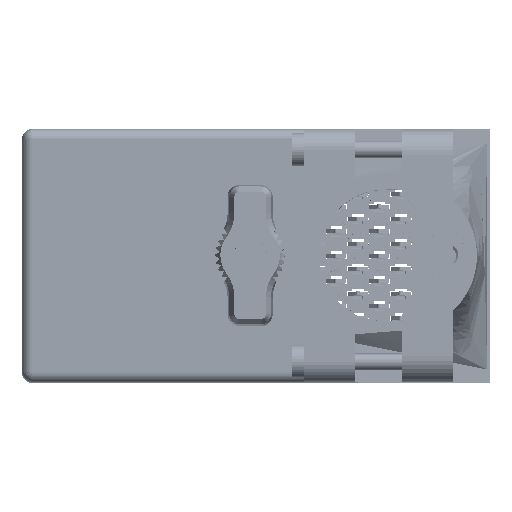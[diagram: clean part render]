
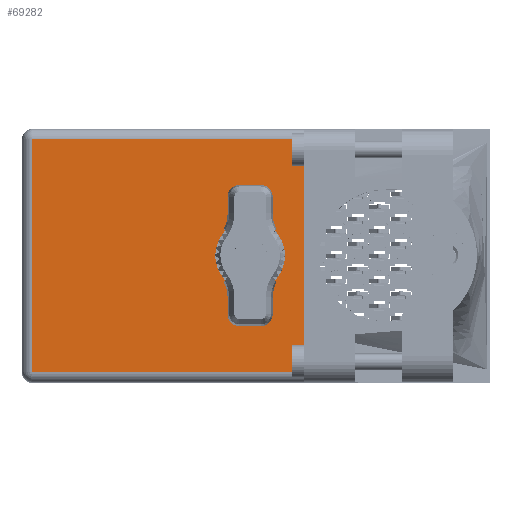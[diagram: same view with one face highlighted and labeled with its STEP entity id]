
A CAD part, top view. The second image highlights one B-rep face of the part: STEP entity #69282.
In plain terms, the highlighted face is planar.
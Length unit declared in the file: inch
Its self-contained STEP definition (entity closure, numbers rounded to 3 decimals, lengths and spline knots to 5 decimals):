
#1304 = ORIENTED_EDGE ( 'NONE', *, *, #88833, .F. ) ;
#4832 = DIRECTION ( 'NONE',  ( 0., 1., 0. ) ) ;
#9601 = VECTOR ( 'NONE', #106246, 39.37008 ) ;
#10069 = EDGE_CURVE ( 'NONE', #51063, #36797, #83982, .T. ) ;
#12342 = DIRECTION ( 'NONE',  ( 0., 1., 0. ) ) ;
#13008 = DIRECTION ( 'NONE',  ( 0., 0., 1. ) ) ;
#14986 = VERTEX_POINT ( 'NONE', #34446 ) ;
#15195 = CARTESIAN_POINT ( 'NONE',  ( 0., 1.93, -0.17 ) ) ;
#22111 = AXIS2_PLACEMENT_3D ( 'NONE', #31059, #4832, #13008 ) ;
#22613 = ORIENTED_EDGE ( 'NONE', *, *, #36865, .T. ) ;
#22828 = CARTESIAN_POINT ( 'NONE',  ( -1.3775, 1.93, -0.703 ) ) ;
#27226 = DIRECTION ( 'NONE',  ( 0., 0., 1. ) ) ;
#31059 = CARTESIAN_POINT ( 'NONE',  ( 0., 1.93, 0. ) ) ;
#33357 = EDGE_CURVE ( 'NONE', #52219, #81480, #93656, .T. ) ;
#34446 = CARTESIAN_POINT ( 'NONE',  ( 0.3275, 1.93, 0.703 ) ) ;
#34911 = VECTOR ( 'NONE', #67939, 39.37008 ) ;
#35451 = EDGE_LOOP ( 'NONE', ( #1304, #92665 ) ) ;
#36797 = VERTEX_POINT ( 'NONE', #104232 ) ;
#36865 = EDGE_CURVE ( 'NONE', #115911, #14986, #96219, .T. ) ;
#40876 = CIRCLE ( 'NONE', #74702, 0.17 ) ;
#41959 = DIRECTION ( 'NONE',  ( 1., 0., 0. ) ) ;
#43500 = ORIENTED_EDGE ( 'NONE', *, *, #45026, .T. ) ;
#45026 = EDGE_CURVE ( 'NONE', #81480, #115911, #51684, .T. ) ;
#45258 = DIRECTION ( 'NONE',  ( 0., 1., 0. ) ) ;
#48492 = VECTOR ( 'NONE', #107899, 39.37008 ) ;
#51063 = VERTEX_POINT ( 'NONE', #15195 ) ;
#51684 = LINE ( 'NONE', #105497, #9601 ) ;
#52219 = VERTEX_POINT ( 'NONE', #72164 ) ;
#55409 = AXIS2_PLACEMENT_3D ( 'NONE', #84063, #12342, #75034 ) ;
#55455 = FACE_BOUND ( 'NONE', #35451, .T. ) ;
#63740 = CARTESIAN_POINT ( 'NONE',  ( 0.3275, 1.93, -0.765 ) ) ;
#67939 = DIRECTION ( 'NONE',  ( -1., 0., 0. ) ) ;
#69282 = ADVANCED_FACE ( 'NONE', ( #79278, #55455 ), #75411, .T. ) ;
#72164 = CARTESIAN_POINT ( 'NONE',  ( 0.3275, 1.93, -0.703 ) ) ;
#74702 = AXIS2_PLACEMENT_3D ( 'NONE', #88771, #45258, #27226 ) ;
#75034 = DIRECTION ( 'NONE',  ( -1., 0., 0. ) ) ;
#75411 = PLANE ( 'NONE',  #55409 ) ;
#78103 = EDGE_LOOP ( 'NONE', ( #43500, #22613, #99815, #103140 ) ) ;
#79278 = FACE_OUTER_BOUND ( 'NONE', #78103, .T. ) ;
#80683 = LINE ( 'NONE', #63740, #48492 ) ;
#81480 = VERTEX_POINT ( 'NONE', #88573 ) ;
#83982 = CIRCLE ( 'NONE', #22111, 0.17 ) ;
#84063 = CARTESIAN_POINT ( 'NONE',  ( -1.3775, 1.93, -0.765 ) ) ;
#84764 = EDGE_CURVE ( 'NONE', #52219, #14986, #80683, .T. ) ;
#85877 = CARTESIAN_POINT ( 'NONE',  ( 0.3275, 1.93, 0.703 ) ) ;
#88573 = CARTESIAN_POINT ( 'NONE',  ( -1.3155, 1.93, -0.703 ) ) ;
#88771 = CARTESIAN_POINT ( 'NONE',  ( 0., 1.93, 0. ) ) ;
#88833 = EDGE_CURVE ( 'NONE', #36797, #51063, #40876, .T. ) ;
#92665 = ORIENTED_EDGE ( 'NONE', *, *, #10069, .F. ) ;
#93656 = LINE ( 'NONE', #22828, #34911 ) ;
#96219 = LINE ( 'NONE', #85877, #99016 ) ;
#99016 = VECTOR ( 'NONE', #41959, 39.37008 ) ;
#99815 = ORIENTED_EDGE ( 'NONE', *, *, #84764, .F. ) ;
#103140 = ORIENTED_EDGE ( 'NONE', *, *, #33357, .T. ) ;
#104232 = CARTESIAN_POINT ( 'NONE',  ( 0., 1.93, 0.17 ) ) ;
#105497 = CARTESIAN_POINT ( 'NONE',  ( -1.3155, 1.93, -0.765 ) ) ;
#106246 = DIRECTION ( 'NONE',  ( 0., 0., 1. ) ) ;
#107899 = DIRECTION ( 'NONE',  ( 0., 0., 1. ) ) ;
#114450 = CARTESIAN_POINT ( 'NONE',  ( -1.3155, 1.93, 0.703 ) ) ;
#115911 = VERTEX_POINT ( 'NONE', #114450 ) ;
